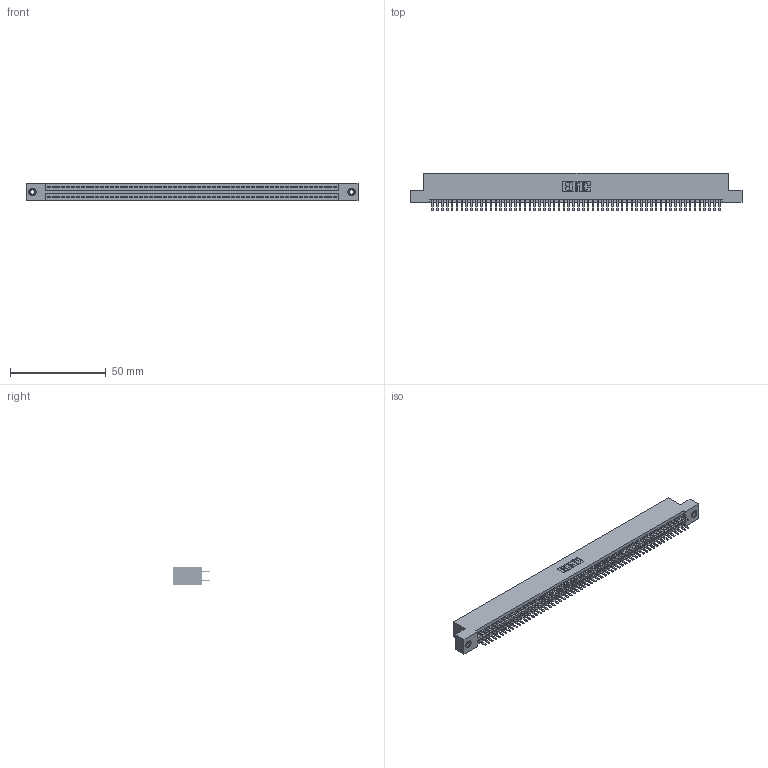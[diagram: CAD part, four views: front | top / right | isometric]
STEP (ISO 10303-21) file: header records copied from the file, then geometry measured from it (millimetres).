
FILE_DESCRIPTION (( 'STEP AP203' ), '1' );
FILE_NAME ('845-120-520-208.STEP', '2018-11-21T01:04:10', ( '' ), ( '' ), 'SwSTEP 2.0', 'SolidWorks 2016', '' );
FILE_SCHEMA (( 'CONFIG_CONTROL_DESIGN' ));
Length unit declared in the file: inch
Products named in the file (4): 345-292-001_345-293-120; 345-250-001_345-250-003-102; 845-120-520-208; 845 Part_Flush Mounting Lugs - 0.156 Dia-TI
Assembly tree (123 placements, depth 2):
  845-120-520-208
    845 Part_Flush Mounting Lugs - 0.156 Dia-TI
    345-292-001_345-293-120  x120
    345-250-001_345-250-003-102  x2
Bounding box: 173.61 x 19.68 x 9.4 mm (x, y, z)
Volume: 16972.4 mm3; surface area: 25337.9 mm2
Topology: 123 solids, 123 shells, 6666 faces, 19317 edges, 12550 vertices
Faces by surface type: plane 4312, cylinder 2338, cone 12, torus 4
Entity records: 45954 total; most frequent: CARTESIAN_POINT 7679, ORIENTED_EDGE 7594, DIRECTION 6763, EDGE_CURVE 3797, LINE 3401, VECTOR 3401, VERTEX_POINT 2524, AXIS2_PLACEMENT_3D 1681
